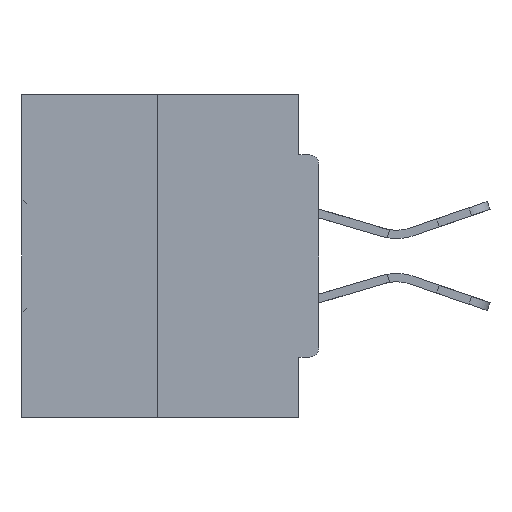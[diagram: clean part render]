
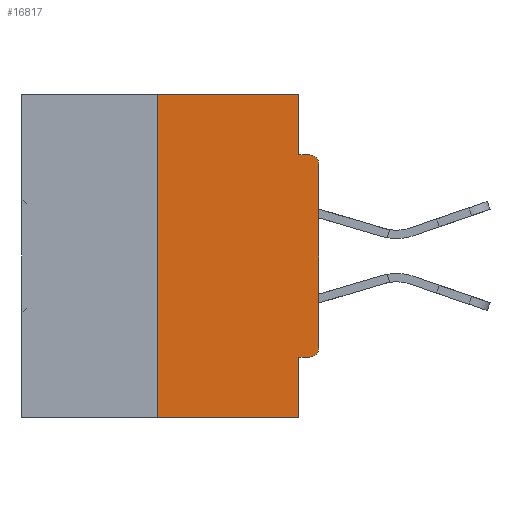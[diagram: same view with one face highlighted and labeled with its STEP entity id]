
A CAD part, left-side view. The second image highlights one B-rep face of the part: STEP entity #16817.
In plain terms, the highlighted planar face has unit normal (-1, 0, 0).
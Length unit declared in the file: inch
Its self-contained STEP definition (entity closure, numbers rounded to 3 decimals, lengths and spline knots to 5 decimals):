
#608 = EDGE_LOOP ( 'NONE', ( #38140, #10464, #13463, #44834, #23388, #10029, #17247, #30526, #9673, #9918 ) ) ;
#622 = DIRECTION ( 'NONE',  ( 0., 0., -1. ) ) ;
#2970 = VECTOR ( 'NONE', #16945, 39.37008 ) ;
#4418 = EDGE_CURVE ( 'NONE', #10557, #29816, #15225, .T. ) ;
#4817 = CARTESIAN_POINT ( 'NONE',  ( 0., 0.015, -0.3915 ) ) ;
#4889 = VERTEX_POINT ( 'NONE', #39728 ) ;
#5081 = EDGE_CURVE ( 'NONE', #34545, #35833, #24788, .T. ) ;
#6220 = DIRECTION ( 'NONE',  ( 0., 0., 1. ) ) ;
#6252 = VECTOR ( 'NONE', #45289, 39.37008 ) ;
#6784 = CARTESIAN_POINT ( 'NONE',  ( 0., 0.46, -0.5 ) ) ;
#7460 = DIRECTION ( 'NONE',  ( 0., 0., -1. ) ) ;
#8225 = EDGE_CURVE ( 'NONE', #25104, #39232, #42956, .T. ) ;
#9673 = ORIENTED_EDGE ( 'NONE', *, *, #45803, .F. ) ;
#9918 = ORIENTED_EDGE ( 'NONE', *, *, #8225, .F. ) ;
#10029 = ORIENTED_EDGE ( 'NONE', *, *, #26121, .T. ) ;
#10450 = CARTESIAN_POINT ( 'NONE',  ( 0., 0., -0.1085 ) ) ;
#10464 = ORIENTED_EDGE ( 'NONE', *, *, #29158, .F. ) ;
#10557 = VERTEX_POINT ( 'NONE', #28297 ) ;
#11374 = CARTESIAN_POINT ( 'NONE',  ( 0., 0.031, -0.4065 ) ) ;
#11491 = CARTESIAN_POINT ( 'NONE',  ( 0., 0.031, 0. ) ) ;
#11506 = LINE ( 'NONE', #25612, #38995 ) ;
#12196 = VERTEX_POINT ( 'NONE', #36224 ) ;
#13083 = CARTESIAN_POINT ( 'NONE',  ( 0., 0.25, 0. ) ) ;
#13323 = VERTEX_POINT ( 'NONE', #45064 ) ;
#13463 = ORIENTED_EDGE ( 'NONE', *, *, #4418, .T. ) ;
#14887 = VECTOR ( 'NONE', #7460, 39.37008 ) ;
#14994 = AXIS2_PLACEMENT_3D ( 'NONE', #29017, #39508, #36396 ) ;
#15225 = LINE ( 'NONE', #6784, #2970 ) ;
#15620 = VECTOR ( 'NONE', #25813, 39.37008 ) ;
#16223 = AXIS2_PLACEMENT_3D ( 'NONE', #38072, #27243, #20031 ) ;
#16817 = ADVANCED_FACE ( 'NONE', ( #38430 ), #34434, .F. ) ;
#16945 = DIRECTION ( 'NONE',  ( 0., -1., 0. ) ) ;
#17247 = ORIENTED_EDGE ( 'NONE', *, *, #43551, .T. ) ;
#20031 = DIRECTION ( 'NONE',  ( 0., 0., -1. ) ) ;
#22980 = DIRECTION ( 'NONE',  ( 0., 0., -1. ) ) ;
#23388 = ORIENTED_EDGE ( 'NONE', *, *, #5081, .F. ) ;
#24436 = LINE ( 'NONE', #13083, #38966 ) ;
#24709 = CIRCLE ( 'NONE', #14994, 0.015 ) ;
#24788 = LINE ( 'NONE', #30471, #6252 ) ;
#25104 = VERTEX_POINT ( 'NONE', #44902 ) ;
#25612 = CARTESIAN_POINT ( 'NONE',  ( 0., 0., -0.0935 ) ) ;
#25813 = DIRECTION ( 'NONE',  ( 0., 0., 1. ) ) ;
#26119 = CARTESIAN_POINT ( 'NONE',  ( 0., 0.031, -0.5 ) ) ;
#26121 = EDGE_CURVE ( 'NONE', #34545, #12196, #28883, .T. ) ;
#26642 = VECTOR ( 'NONE', #36678, 39.37008 ) ;
#27243 = DIRECTION ( 'NONE',  ( 1., 0., 0. ) ) ;
#28000 = CARTESIAN_POINT ( 'NONE',  ( 0., 0.031, -0.0935 ) ) ;
#28297 = CARTESIAN_POINT ( 'NONE',  ( 0., 0.25, -0.5 ) ) ;
#28883 = CIRCLE ( 'NONE', #45885, 0.015 ) ;
#29017 = CARTESIAN_POINT ( 'NONE',  ( 0., 0.015, -0.1085 ) ) ;
#29158 = EDGE_CURVE ( 'NONE', #10557, #13323, #24436, .T. ) ;
#29396 = LINE ( 'NONE', #43899, #26642 ) ;
#29628 = LINE ( 'NONE', #36045, #40235 ) ;
#29816 = VERTEX_POINT ( 'NONE', #26119 ) ;
#30471 = CARTESIAN_POINT ( 'NONE',  ( 0., 0., -0.4065 ) ) ;
#30526 = ORIENTED_EDGE ( 'NONE', *, *, #42790, .T. ) ;
#31398 = CARTESIAN_POINT ( 'NONE',  ( 0., 0.015, -0.4065 ) ) ;
#32723 = CARTESIAN_POINT ( 'NONE',  ( 0., 0., 0. ) ) ;
#33693 = EDGE_CURVE ( 'NONE', #35833, #29816, #29628, .T. ) ;
#34139 = LINE ( 'NONE', #32723, #15620 ) ;
#34434 = PLANE ( 'NONE',  #16223 ) ;
#34545 = VERTEX_POINT ( 'NONE', #31398 ) ;
#35833 = VERTEX_POINT ( 'NONE', #11374 ) ;
#36045 = CARTESIAN_POINT ( 'NONE',  ( 0., 0.031, -0.5 ) ) ;
#36224 = CARTESIAN_POINT ( 'NONE',  ( 0., 0., -0.3915 ) ) ;
#36283 = DIRECTION ( 'NONE',  ( 0., -1., 0. ) ) ;
#36396 = DIRECTION ( 'NONE',  ( 0., 0., -1. ) ) ;
#36678 = DIRECTION ( 'NONE',  ( 0., -1., 0. ) ) ;
#38072 = CARTESIAN_POINT ( 'NONE',  ( 0., 0.46, 0. ) ) ;
#38140 = ORIENTED_EDGE ( 'NONE', *, *, #46086, .F. ) ;
#38430 = FACE_OUTER_BOUND ( 'NONE', #608, .T. ) ;
#38966 = VECTOR ( 'NONE', #6220, 39.37008 ) ;
#38995 = VECTOR ( 'NONE', #36283, 39.37008 ) ;
#39232 = VERTEX_POINT ( 'NONE', #28000 ) ;
#39508 = DIRECTION ( 'NONE',  ( -1., 0., 0. ) ) ;
#39728 = CARTESIAN_POINT ( 'NONE',  ( 0., 0.015, -0.0935 ) ) ;
#40235 = VECTOR ( 'NONE', #622, 39.37008 ) ;
#40382 = DIRECTION ( 'NONE',  ( -1., 0., 0. ) ) ;
#42790 = EDGE_CURVE ( 'NONE', #43971, #4889, #24709, .T. ) ;
#42956 = LINE ( 'NONE', #11491, #14887 ) ;
#43551 = EDGE_CURVE ( 'NONE', #12196, #43971, #34139, .T. ) ;
#43899 = CARTESIAN_POINT ( 'NONE',  ( 0., 0.46, 0. ) ) ;
#43971 = VERTEX_POINT ( 'NONE', #10450 ) ;
#44834 = ORIENTED_EDGE ( 'NONE', *, *, #33693, .F. ) ;
#44902 = CARTESIAN_POINT ( 'NONE',  ( 0., 0.031, 0. ) ) ;
#45064 = CARTESIAN_POINT ( 'NONE',  ( 0., 0.25, 0. ) ) ;
#45289 = DIRECTION ( 'NONE',  ( 0., 1., 0. ) ) ;
#45803 = EDGE_CURVE ( 'NONE', #39232, #4889, #11506, .T. ) ;
#45885 = AXIS2_PLACEMENT_3D ( 'NONE', #4817, #40382, #22980 ) ;
#46086 = EDGE_CURVE ( 'NONE', #13323, #25104, #29396, .T. ) ;
